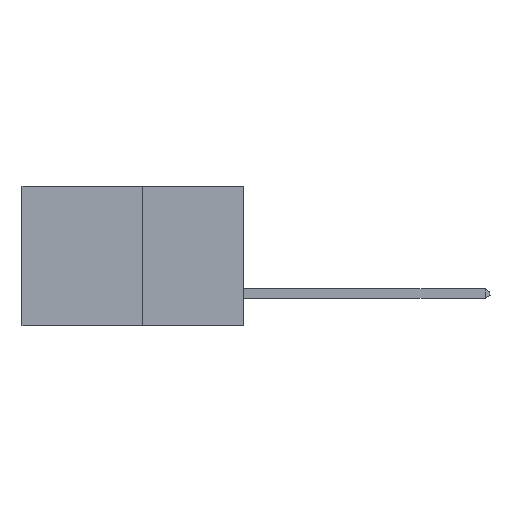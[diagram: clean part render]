
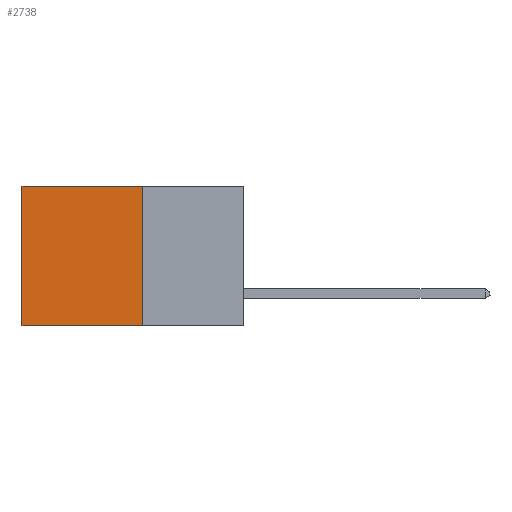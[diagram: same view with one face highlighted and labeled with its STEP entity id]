
A CAD part, left-side view. The second image highlights one B-rep face of the part: STEP entity #2738.
In plain terms, the highlighted planar face has unit normal (-1, 0, 0).
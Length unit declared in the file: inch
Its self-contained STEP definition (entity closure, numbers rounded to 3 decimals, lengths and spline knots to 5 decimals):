
#520 = VERTEX_POINT ( 'NONE', #664 ) ;
#664 = CARTESIAN_POINT ( 'NONE',  ( 0.277, 0.59, 0. ) ) ;
#900 = ORIENTED_EDGE ( 'NONE', *, *, #8634, .T. ) ;
#1277 = DIRECTION ( 'NONE',  ( 0., 0., -1. ) ) ;
#1317 = VECTOR ( 'NONE', #1769, 39.37008 ) ;
#1516 = VECTOR ( 'NONE', #10444, 39.37008 ) ;
#1769 = DIRECTION ( 'NONE',  ( 0., 0., -1. ) ) ;
#1839 = LINE ( 'NONE', #11011, #1516 ) ;
#1885 = VECTOR ( 'NONE', #9234, 39.37008 ) ;
#2383 = EDGE_LOOP ( 'NONE', ( #900, #4991, #10673, #3927 ) ) ;
#2738 = ADVANCED_FACE ( 'NONE', ( #11328 ), #5160, .F. ) ;
#3695 = EDGE_CURVE ( 'NONE', #4211, #4395, #4272, .T. ) ;
#3927 = ORIENTED_EDGE ( 'NONE', *, *, #7559, .T. ) ;
#4211 = VERTEX_POINT ( 'NONE', #9235 ) ;
#4272 = LINE ( 'NONE', #5667, #1885 ) ;
#4384 = CARTESIAN_POINT ( 'NONE',  ( 0.277, 0.27, 0. ) ) ;
#4395 = VERTEX_POINT ( 'NONE', #9400 ) ;
#4628 = DIRECTION ( 'NONE',  ( 0., 1., 0. ) ) ;
#4991 = ORIENTED_EDGE ( 'NONE', *, *, #3695, .F. ) ;
#5160 = PLANE ( 'NONE',  #6802 ) ;
#5667 = CARTESIAN_POINT ( 'NONE',  ( 0.277, 0.27, -0.37 ) ) ;
#5674 = VECTOR ( 'NONE', #4628, 39.37008 ) ;
#6802 = AXIS2_PLACEMENT_3D ( 'NONE', #11082, #10954, #1277 ) ;
#7262 = EDGE_CURVE ( 'NONE', #11867, #4211, #1839, .T. ) ;
#7559 = EDGE_CURVE ( 'NONE', #11867, #520, #10832, .T. ) ;
#8555 = CARTESIAN_POINT ( 'NONE',  ( 0.277, 0.59, -0.37 ) ) ;
#8634 = EDGE_CURVE ( 'NONE', #520, #4395, #8760, .T. ) ;
#8760 = LINE ( 'NONE', #8555, #1317 ) ;
#9234 = DIRECTION ( 'NONE',  ( 0., 1., 0. ) ) ;
#9235 = CARTESIAN_POINT ( 'NONE',  ( 0.277, 0.27, -0.37 ) ) ;
#9400 = CARTESIAN_POINT ( 'NONE',  ( 0.277, 0.59, -0.37 ) ) ;
#10383 = CARTESIAN_POINT ( 'NONE',  ( 0.277, 0.27, 0. ) ) ;
#10444 = DIRECTION ( 'NONE',  ( 0., 0., -1. ) ) ;
#10673 = ORIENTED_EDGE ( 'NONE', *, *, #7262, .F. ) ;
#10832 = LINE ( 'NONE', #4384, #5674 ) ;
#10954 = DIRECTION ( 'NONE',  ( 1., 0., 0. ) ) ;
#11011 = CARTESIAN_POINT ( 'NONE',  ( 0.277, 0.27, -0.37 ) ) ;
#11082 = CARTESIAN_POINT ( 'NONE',  ( 0.277, 0.27, -0.37 ) ) ;
#11328 = FACE_OUTER_BOUND ( 'NONE', #2383, .T. ) ;
#11867 = VERTEX_POINT ( 'NONE', #10383 ) ;
